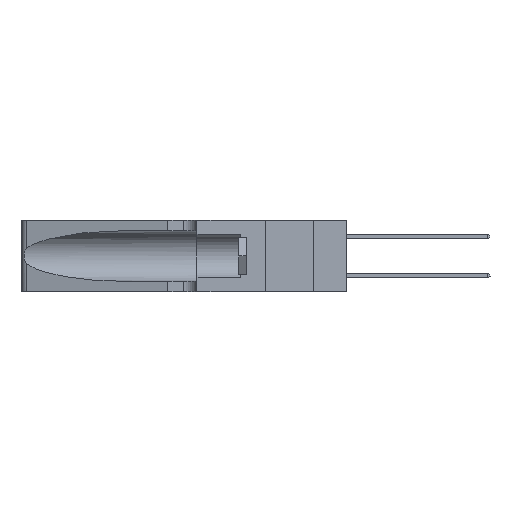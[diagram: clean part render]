
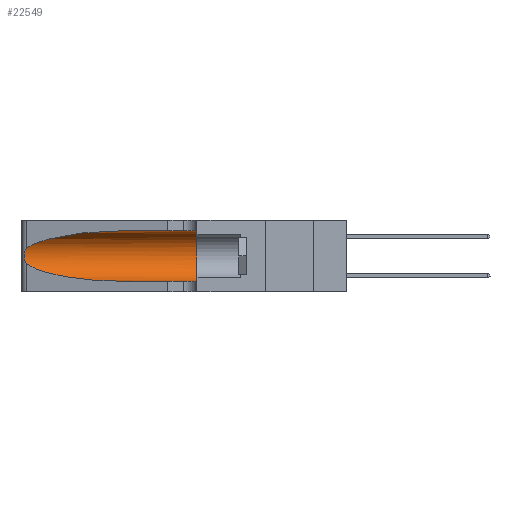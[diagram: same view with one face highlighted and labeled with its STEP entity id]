
A CAD part, left-side view. The second image highlights one B-rep face of the part: STEP entity #22549.
In plain terms, the highlighted cylindrical face has radius 3.308 mm (diameter 6.617 mm), a partial arc.
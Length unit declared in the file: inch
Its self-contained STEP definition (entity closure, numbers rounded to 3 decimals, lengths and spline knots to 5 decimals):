
#1028 = CARTESIAN_POINT ( 'NONE',  ( 0.26018, 1.23835, 0.19895 ) ) ;
#1128 = EDGE_CURVE ( 'NONE', #5067, #32908, #22560, .T. ) ;
#1474 = CARTESIAN_POINT ( 'NONE',  ( 0.25487, 1.22718, 0.14631 ) ) ;
#2253 = EDGE_CURVE ( 'NONE', #32908, #18850, #27938, .T. ) ;
#2851 = EDGE_CURVE ( 'NONE', #10545, #18850, #22397, .T. ) ;
#4475 = AXIS2_PLACEMENT_3D ( 'NONE', #16032, #16738, #26368 ) ;
#4639 = ORIENTED_EDGE ( 'NONE', *, *, #30759, .T. ) ;
#5067 = VERTEX_POINT ( 'NONE', #33611 ) ;
#6772 =( BOUNDED_CURVE ( )  B_SPLINE_CURVE ( 3, ( #37394, #24745, #37262, #21705 ),
 .UNSPECIFIED., .F., .T. ) 
 B_SPLINE_CURVE_WITH_KNOTS ( ( 4, 4 ),
 ( 3.44316, 4.71239 ),
 .UNSPECIFIED. ) 
 CURVE ( )  GEOMETRIC_REPRESENTATION_ITEM ( )  RATIONAL_B_SPLINE_CURVE ( ( 1., 0.87, 0.87, 1. ) ) 
 REPRESENTATION_ITEM ( '' )  );
#7009 = CARTESIAN_POINT ( 'NONE',  ( 0.26075, 1.23896, 0.178 ) ) ;
#7268 = CARTESIAN_POINT ( 'NONE',  ( 0.1305, 0.72297, 0.31525 ) ) ;
#7580 = CARTESIAN_POINT ( 'NONE',  ( 0.26075, 1.23896, 0.19203 ) ) ;
#9199 = ORIENTED_EDGE ( 'NONE', *, *, #32161, .T. ) ;
#9798 = VECTOR ( 'NONE', #20319, 39.37008 ) ;
#10322 = CARTESIAN_POINT ( 'NONE',  ( 0.25487, 1.22718, 0.22369 ) ) ;
#10545 = VERTEX_POINT ( 'NONE', #36114 ) ;
#10671 = CARTESIAN_POINT ( 'NONE',  ( 0.1305, 0.35, 0.185 ) ) ;
#10840 = ORIENTED_EDGE ( 'NONE', *, *, #23915, .T. ) ;
#12990 = VERTEX_POINT ( 'NONE', #38617 ) ;
#13449 = CARTESIAN_POINT ( 'NONE',  ( 0.26017, 1.23833, 0.17102 ) ) ;
#13589 = CARTESIAN_POINT ( 'NONE',  ( 0.1305, 1.61858, 0.31525 ) ) ;
#13886 = CARTESIAN_POINT ( 'NONE',  ( 0.25854, 1.2359, 0.20912 ) ) ;
#14837 =( BOUNDED_CURVE ( )  B_SPLINE_CURVE ( 3, ( #7268, #16876, #19602, #10322 ),
 .UNSPECIFIED., .F., .T. ) 
 B_SPLINE_CURVE_WITH_KNOTS ( ( 4, 4 ),
 ( 1.5708, 2.84003 ),
 .UNSPECIFIED. ) 
 CURVE ( )  GEOMETRIC_REPRESENTATION_ITEM ( )  RATIONAL_B_SPLINE_CURVE ( ( 1., 0.87, 0.87, 1. ) ) 
 REPRESENTATION_ITEM ( '' )  );
#15990 = VERTEX_POINT ( 'NONE', #37158 ) ;
#16032 = CARTESIAN_POINT ( 'NONE',  ( 0.1305, 1.61858, 0.185 ) ) ;
#16154 = ORIENTED_EDGE ( 'NONE', *, *, #2851, .T. ) ;
#16738 = DIRECTION ( 'NONE',  ( 0., -1., 0. ) ) ;
#16876 = CARTESIAN_POINT ( 'NONE',  ( 0.18966, 0.96281, 0.31525 ) ) ;
#17014 = VECTOR ( 'NONE', #25908, 39.37008 ) ;
#17905 = AXIS2_PLACEMENT_3D ( 'NONE', #10671, #39932, #23240 ) ;
#18850 = VERTEX_POINT ( 'NONE', #19690 ) ;
#19602 = CARTESIAN_POINT ( 'NONE',  ( 0.2373, 1.15595, 0.28018 ) ) ;
#19690 = CARTESIAN_POINT ( 'NONE',  ( 0.1305, 0.35, 0.05475 ) ) ;
#19722 = ORIENTED_EDGE ( 'NONE', *, *, #2253, .F. ) ;
#20319 = DIRECTION ( 'NONE',  ( 0., -1., 0. ) ) ;
#21705 = CARTESIAN_POINT ( 'NONE',  ( 0.1305, 0.72297, 0.05475 ) ) ;
#21794 = CARTESIAN_POINT ( 'NONE',  ( 0.1305, 0.35, 0.31525 ) ) ;
#22397 = LINE ( 'NONE', #22752, #17014 ) ;
#22549 = ADVANCED_FACE ( 'NONE', ( #23764 ), #30126, .F. ) ;
#22560 = LINE ( 'NONE', #13589, #9798 ) ;
#22752 = CARTESIAN_POINT ( 'NONE',  ( 0.1305, 1.61858, 0.05475 ) ) ;
#23094 = CARTESIAN_POINT ( 'NONE',  ( 0.25856, 1.23593, 0.16098 ) ) ;
#23240 = DIRECTION ( 'NONE',  ( 0., 0., 1. ) ) ;
#23764 = FACE_OUTER_BOUND ( 'NONE', #31980, .T. ) ;
#23915 = EDGE_CURVE ( 'NONE', #5067, #15990, #14837, .T. ) ;
#24745 = CARTESIAN_POINT ( 'NONE',  ( 0.2373, 1.15595, 0.08982 ) ) ;
#25313 = CARTESIAN_POINT ( 'NONE',  ( 0.25639, 1.23184, 0.21858 ) ) ;
#25826 = CARTESIAN_POINT ( 'NONE',  ( 0.25787, 1.23484, 0.2124 ) ) ;
#25908 = DIRECTION ( 'NONE',  ( 0., -1., 0. ) ) ;
#25977 = CARTESIAN_POINT ( 'NONE',  ( 0.25639, 1.23186, 0.15144 ) ) ;
#26368 = DIRECTION ( 'NONE',  ( 0., 0., -1. ) ) ;
#27938 = CIRCLE ( 'NONE', #17905, 0.13025 ) ;
#30126 = CYLINDRICAL_SURFACE ( 'NONE', #4475, 0.13025 ) ;
#30759 = EDGE_CURVE ( 'NONE', #15990, #12990, #36636, .T. ) ;
#31980 = EDGE_LOOP ( 'NONE', ( #10840, #4639, #9199, #16154, #19722, #34746 ) ) ;
#32133 = CARTESIAN_POINT ( 'NONE',  ( 0.25555, 1.22993, 0.14849 ) ) ;
#32161 = EDGE_CURVE ( 'NONE', #12990, #10545, #6772, .T. ) ;
#32542 = CARTESIAN_POINT ( 'NONE',  ( 0.25789, 1.23486, 0.15765 ) ) ;
#32908 = VERTEX_POINT ( 'NONE', #21794 ) ;
#33611 = CARTESIAN_POINT ( 'NONE',  ( 0.1305, 0.72297, 0.31525 ) ) ;
#34746 = ORIENTED_EDGE ( 'NONE', *, *, #1128, .F. ) ;
#35069 = CARTESIAN_POINT ( 'NONE',  ( 0.25555, 1.22994, 0.2215 ) ) ;
#36114 = CARTESIAN_POINT ( 'NONE',  ( 0.1305, 0.72297, 0.05475 ) ) ;
#36636 = B_SPLINE_CURVE_WITH_KNOTS ( 'NONE', 3,
 ( #37936, #35069, #25313, #25826, #13886, #1028, #7580, #7009, #13449, #23094, #32542, #25977, #32133, #1474 ),
 .UNSPECIFIED., .F., .F.,
 ( 4, 2, 2, 2, 2, 2, 4 ),
 ( 0., 0.00027, 0.00053, 0.00107, 0.0016, 0.00187, 0.00214 ),
 .UNSPECIFIED. ) ;
#37158 = CARTESIAN_POINT ( 'NONE',  ( 0.25487, 1.22718, 0.22369 ) ) ;
#37262 = CARTESIAN_POINT ( 'NONE',  ( 0.18966, 0.96281, 0.05475 ) ) ;
#37394 = CARTESIAN_POINT ( 'NONE',  ( 0.25487, 1.22718, 0.14631 ) ) ;
#37936 = CARTESIAN_POINT ( 'NONE',  ( 0.25487, 1.22718, 0.22369 ) ) ;
#38617 = CARTESIAN_POINT ( 'NONE',  ( 0.25487, 1.22718, 0.14631 ) ) ;
#39932 = DIRECTION ( 'NONE',  ( 0., 1., 0. ) ) ;
